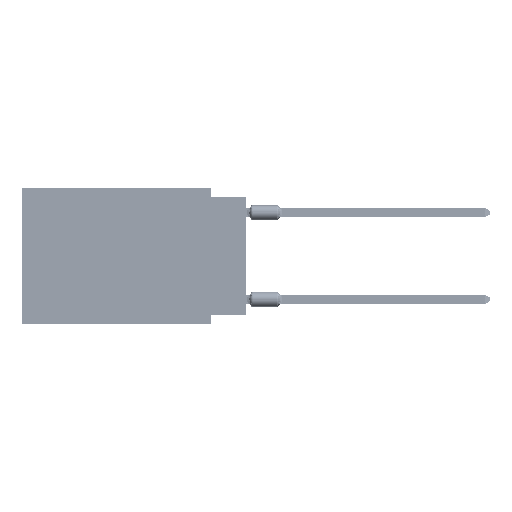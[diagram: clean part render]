
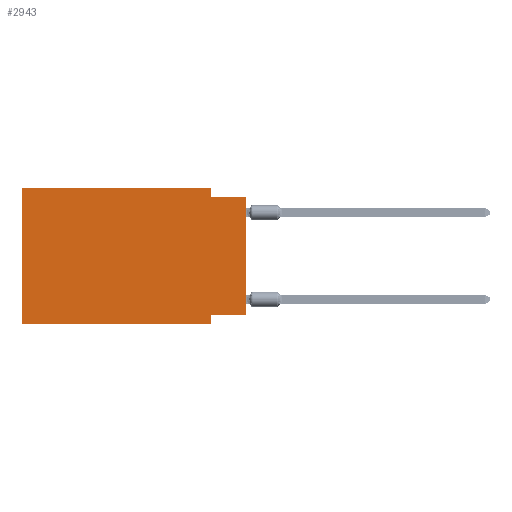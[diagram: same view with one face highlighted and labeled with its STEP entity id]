
A CAD part, left-side view. The second image highlights one B-rep face of the part: STEP entity #2943.
In plain terms, the highlighted planar face has unit normal (-1, 0, 0).
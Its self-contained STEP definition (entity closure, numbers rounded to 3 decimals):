
#2943 = ADVANCED_FACE ( 'NONE', ( #85099 ), #8892, .F. ) ;
#5075 = CARTESIAN_POINT ( 'NONE',  ( 0., 2.54, 0. ) ) ;
#6187 = DIRECTION ( 'NONE',  ( 0., 0., -1. ) ) ;
#7144 = CARTESIAN_POINT ( 'NONE',  ( 0., 0., -0.635 ) ) ;
#8892 = PLANE ( 'NONE',  #31847 ) ;
#9310 = VERTEX_POINT ( 'NONE', #34719 ) ;
#10382 = EDGE_CURVE ( 'NONE', #17121, #14019, #26046, .T. ) ;
#11150 = EDGE_CURVE ( 'NONE', #52069, #36811, #17798, .T. ) ;
#13572 = EDGE_CURVE ( 'NONE', #36811, #80412, #38617, .T. ) ;
#14019 = VERTEX_POINT ( 'NONE', #7144 ) ;
#14252 = ORIENTED_EDGE ( 'NONE', *, *, #10382, .T. ) ;
#14320 = DIRECTION ( 'NONE',  ( 0., 0., -1. ) ) ;
#14817 = VECTOR ( 'NONE', #14320, 1000. ) ;
#15136 = CARTESIAN_POINT ( 'NONE',  ( 0., 0., -0.635 ) ) ;
#15709 = EDGE_CURVE ( 'NONE', #9310, #22744, #75437, .T. ) ;
#15765 = DIRECTION ( 'NONE',  ( 0., 1., 0. ) ) ;
#16813 = ORIENTED_EDGE ( 'NONE', *, *, #13572, .F. ) ;
#17121 = VERTEX_POINT ( 'NONE', #46182 ) ;
#17798 = LINE ( 'NONE', #31048, #49738 ) ;
#19658 = ORIENTED_EDGE ( 'NONE', *, *, #52611, .T. ) ;
#22612 = DIRECTION ( 'NONE',  ( 0., -1., 0. ) ) ;
#22744 = VERTEX_POINT ( 'NONE', #84730 ) ;
#23284 = ORIENTED_EDGE ( 'NONE', *, *, #11150, .F. ) ;
#24671 = VECTOR ( 'NONE', #15765, 1000. ) ;
#26046 = LINE ( 'NONE', #65783, #54102 ) ;
#31048 = CARTESIAN_POINT ( 'NONE',  ( 0., 16.383, 0. ) ) ;
#31291 = VECTOR ( 'NONE', #57425, 1000. ) ;
#31847 = AXIS2_PLACEMENT_3D ( 'NONE', #78032, #44507, #48617 ) ;
#34334 = CARTESIAN_POINT ( 'NONE',  ( 0., 0., -9.271 ) ) ;
#34719 = CARTESIAN_POINT ( 'NONE',  ( 0., 2.54, -9.271 ) ) ;
#36811 = VERTEX_POINT ( 'NONE', #56097 ) ;
#37773 = ORIENTED_EDGE ( 'NONE', *, *, #15709, .F. ) ;
#37906 = CARTESIAN_POINT ( 'NONE',  ( 0., 16.383, -9.906 ) ) ;
#38172 = EDGE_LOOP ( 'NONE', ( #14252, #78550, #16813, #23284, #80621, #19658, #37773, #61449 ) ) ;
#38617 = LINE ( 'NONE', #5075, #14817 ) ;
#38817 = CARTESIAN_POINT ( 'NONE',  ( 0., 2.54, -0.635 ) ) ;
#39218 = DIRECTION ( 'NONE',  ( 0., -1., 0. ) ) ;
#39348 = CARTESIAN_POINT ( 'NONE',  ( 0., 16.383, -9.906 ) ) ;
#41723 = CARTESIAN_POINT ( 'NONE',  ( 0., 16.383, 0. ) ) ;
#42027 = VECTOR ( 'NONE', #6187, 1000. ) ;
#42419 = VECTOR ( 'NONE', #39218, 1000. ) ;
#44507 = DIRECTION ( 'NONE',  ( 1., 0., 0. ) ) ;
#44730 = DIRECTION ( 'NONE',  ( 0., -1., 0. ) ) ;
#45539 = EDGE_CURVE ( 'NONE', #51453, #52069, #70635, .T. ) ;
#46182 = CARTESIAN_POINT ( 'NONE',  ( 0., 0., -9.271 ) ) ;
#48617 = DIRECTION ( 'NONE',  ( 0., 0., -1. ) ) ;
#49264 = EDGE_CURVE ( 'NONE', #17121, #9310, #62134, .T. ) ;
#49738 = VECTOR ( 'NONE', #44730, 1000. ) ;
#51453 = VERTEX_POINT ( 'NONE', #39348 ) ;
#52069 = VERTEX_POINT ( 'NONE', #41723 ) ;
#52611 = EDGE_CURVE ( 'NONE', #51453, #22744, #58674, .T. ) ;
#54102 = VECTOR ( 'NONE', #64908, 1000. ) ;
#54991 = EDGE_CURVE ( 'NONE', #80412, #14019, #82654, .T. ) ;
#55383 = VECTOR ( 'NONE', #22612, 1000. ) ;
#56097 = CARTESIAN_POINT ( 'NONE',  ( 0., 2.54, 0. ) ) ;
#57425 = DIRECTION ( 'NONE',  ( 0., 0., 1. ) ) ;
#58674 = LINE ( 'NONE', #37906, #42419 ) ;
#61449 = ORIENTED_EDGE ( 'NONE', *, *, #49264, .F. ) ;
#62134 = LINE ( 'NONE', #34334, #24671 ) ;
#64908 = DIRECTION ( 'NONE',  ( 0., 0., 1. ) ) ;
#65783 = CARTESIAN_POINT ( 'NONE',  ( 0., 0., 0. ) ) ;
#66648 = CARTESIAN_POINT ( 'NONE',  ( 0., 2.54, -9.906 ) ) ;
#70635 = LINE ( 'NONE', #83018, #31291 ) ;
#75437 = LINE ( 'NONE', #66648, #42027 ) ;
#78032 = CARTESIAN_POINT ( 'NONE',  ( 0., 16.383, 0. ) ) ;
#78550 = ORIENTED_EDGE ( 'NONE', *, *, #54991, .F. ) ;
#80412 = VERTEX_POINT ( 'NONE', #38817 ) ;
#80621 = ORIENTED_EDGE ( 'NONE', *, *, #45539, .F. ) ;
#82654 = LINE ( 'NONE', #15136, #55383 ) ;
#83018 = CARTESIAN_POINT ( 'NONE',  ( 0., 16.383, 0. ) ) ;
#84730 = CARTESIAN_POINT ( 'NONE',  ( 0., 2.54, -9.906 ) ) ;
#85099 = FACE_OUTER_BOUND ( 'NONE', #38172, .T. ) ;
